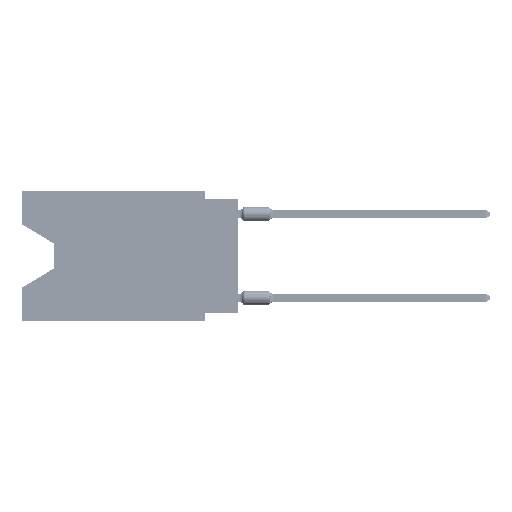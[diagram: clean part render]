
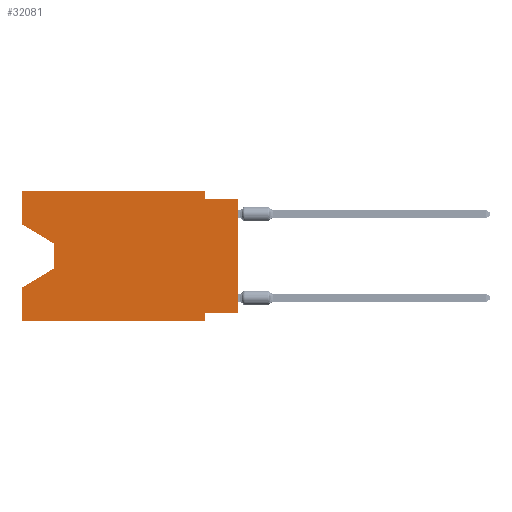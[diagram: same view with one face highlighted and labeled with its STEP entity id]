
A CAD part, left-side view. The second image highlights one B-rep face of the part: STEP entity #32081.
In plain terms, the highlighted planar face has unit normal (-1, 0, 0).
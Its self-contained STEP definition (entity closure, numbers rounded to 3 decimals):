
#15 = CARTESIAN_POINT ( 'NONE',  ( 0., 16.383, -2.546 ) ) ;
#694 = EDGE_CURVE ( 'NONE', #13441, #64532, #63593, .T. ) ;
#866 = VECTOR ( 'NONE', #3840, 1000. ) ;
#1405 = LINE ( 'NONE', #64976, #63932 ) ;
#1498 = DIRECTION ( 'NONE',  ( 0., 1., 0. ) ) ;
#2017 = ORIENTED_EDGE ( 'NONE', *, *, #50201, .F. ) ;
#3273 = ORIENTED_EDGE ( 'NONE', *, *, #44155, .T. ) ;
#3840 = DIRECTION ( 'NONE',  ( 0., 0., -1. ) ) ;
#5650 = DIRECTION ( 'NONE',  ( 0., 0., -1. ) ) ;
#6818 = VERTEX_POINT ( 'NONE', #44249 ) ;
#7020 = CARTESIAN_POINT ( 'NONE',  ( 0., 2.54, 0. ) ) ;
#7268 = CARTESIAN_POINT ( 'NONE',  ( 0., 0., -0.635 ) ) ;
#8455 = ORIENTED_EDGE ( 'NONE', *, *, #694, .T. ) ;
#8976 = VECTOR ( 'NONE', #45054, 1000. ) ;
#9652 = ORIENTED_EDGE ( 'NONE', *, *, #63180, .T. ) ;
#9658 = VERTEX_POINT ( 'NONE', #32526 ) ;
#11703 = DIRECTION ( 'NONE',  ( 0., 0., -1. ) ) ;
#13441 = VERTEX_POINT ( 'NONE', #51184 ) ;
#15927 = VECTOR ( 'NONE', #1498, 1000. ) ;
#16631 = ORIENTED_EDGE ( 'NONE', *, *, #37350, .F. ) ;
#17335 = ORIENTED_EDGE ( 'NONE', *, *, #67220, .F. ) ;
#17505 = LINE ( 'NONE', #7020, #40923 ) ;
#17630 = DIRECTION ( 'NONE',  ( 0., -1., 0. ) ) ;
#18729 = CARTESIAN_POINT ( 'NONE',  ( 0., 0., -0.635 ) ) ;
#19974 = VECTOR ( 'NONE', #42565, 1000. ) ;
#20356 = EDGE_CURVE ( 'NONE', #59912, #29675, #22171, .T. ) ;
#22171 = LINE ( 'NONE', #27079, #57389 ) ;
#23335 = LINE ( 'NONE', #7268, #61497 ) ;
#23520 = VECTOR ( 'NONE', #51082, 1000. ) ;
#23574 = EDGE_CURVE ( 'NONE', #48259, #6818, #59783, .T. ) ;
#24421 = LINE ( 'NONE', #61103, #8976 ) ;
#24930 = VERTEX_POINT ( 'NONE', #28432 ) ;
#25836 = CARTESIAN_POINT ( 'NONE',  ( 0., 13.97, -4.013 ) ) ;
#26499 = LINE ( 'NONE', #58636, #19974 ) ;
#26813 = CARTESIAN_POINT ( 'NONE',  ( 0., 16.383, -7.36 ) ) ;
#27079 = CARTESIAN_POINT ( 'NONE',  ( 0., 16.383, 0. ) ) ;
#27426 = CARTESIAN_POINT ( 'NONE',  ( 0., 2.54, -9.271 ) ) ;
#27497 = VERTEX_POINT ( 'NONE', #41341 ) ;
#27695 = CARTESIAN_POINT ( 'NONE',  ( 0., 0., -9.271 ) ) ;
#28432 = CARTESIAN_POINT ( 'NONE',  ( 0., 2.54, -0.635 ) ) ;
#29599 = ORIENTED_EDGE ( 'NONE', *, *, #56746, .F. ) ;
#29675 = VERTEX_POINT ( 'NONE', #50338 ) ;
#30651 = VERTEX_POINT ( 'NONE', #18729 ) ;
#32081 = ADVANCED_FACE ( 'NONE', ( #33329 ), #64420, .F. ) ;
#32390 = VECTOR ( 'NONE', #53031, 1000. ) ;
#32526 = CARTESIAN_POINT ( 'NONE',  ( 0., 13.97, -5.893 ) ) ;
#33329 = FACE_OUTER_BOUND ( 'NONE', #39149, .T. ) ;
#34933 = DIRECTION ( 'NONE',  ( 0., 0., -1. ) ) ;
#35330 = ORIENTED_EDGE ( 'NONE', *, *, #23574, .F. ) ;
#37350 = EDGE_CURVE ( 'NONE', #48322, #43253, #26499, .T. ) ;
#39149 = EDGE_LOOP ( 'NONE', ( #8455, #64731, #9652, #16631, #3273, #35330, #17335, #54751, #2017, #29599, #65523, #47394 ) ) ;
#39301 = VECTOR ( 'NONE', #53462, 1000. ) ;
#40923 = VECTOR ( 'NONE', #34933, 1000. ) ;
#41341 = CARTESIAN_POINT ( 'NONE',  ( 0., 0., -9.271 ) ) ;
#42565 = DIRECTION ( 'NONE',  ( 0., 0., 1. ) ) ;
#43253 = VERTEX_POINT ( 'NONE', #26813 ) ;
#44155 = EDGE_CURVE ( 'NONE', #48322, #6818, #24421, .T. ) ;
#44249 = CARTESIAN_POINT ( 'NONE',  ( 0., 2.54, -9.906 ) ) ;
#44332 = EDGE_CURVE ( 'NONE', #27497, #30651, #52347, .T. ) ;
#44516 = DIRECTION ( 'NONE',  ( 1., 0., 0. ) ) ;
#45054 = DIRECTION ( 'NONE',  ( 0., -1., 0. ) ) ;
#47394 = ORIENTED_EDGE ( 'NONE', *, *, #66400, .F. ) ;
#48259 = VERTEX_POINT ( 'NONE', #27426 ) ;
#48322 = VERTEX_POINT ( 'NONE', #54993 ) ;
#49310 = AXIS2_PLACEMENT_3D ( 'NONE', #54986, #44516, #11703 ) ;
#50201 = EDGE_CURVE ( 'NONE', #24930, #30651, #23335, .T. ) ;
#50338 = CARTESIAN_POINT ( 'NONE',  ( 0., 2.54, 0. ) ) ;
#50806 = CARTESIAN_POINT ( 'NONE',  ( 0., 13.97, -4.013 ) ) ;
#51082 = DIRECTION ( 'NONE',  ( 0., 0.855, -0.519 ) ) ;
#51184 = CARTESIAN_POINT ( 'NONE',  ( 0., 16.383, -2.546 ) ) ;
#51435 = CARTESIAN_POINT ( 'NONE',  ( 0., 13.97, -5.893 ) ) ;
#52347 = LINE ( 'NONE', #62831, #32390 ) ;
#52383 = LINE ( 'NONE', #25836, #866 ) ;
#53031 = DIRECTION ( 'NONE',  ( 0., 0., 1. ) ) ;
#53462 = DIRECTION ( 'NONE',  ( 0., -0.855, -0.519 ) ) ;
#53672 = CARTESIAN_POINT ( 'NONE',  ( 0., 16.383, 0. ) ) ;
#54189 = CARTESIAN_POINT ( 'NONE',  ( 0., 2.54, -9.906 ) ) ;
#54751 = ORIENTED_EDGE ( 'NONE', *, *, #44332, .T. ) ;
#54986 = CARTESIAN_POINT ( 'NONE',  ( 0., 16.383, 0. ) ) ;
#54993 = CARTESIAN_POINT ( 'NONE',  ( 0., 16.383, -9.906 ) ) ;
#56746 = EDGE_CURVE ( 'NONE', #29675, #24930, #17505, .T. ) ;
#57389 = VECTOR ( 'NONE', #17630, 1000. ) ;
#57691 = LINE ( 'NONE', #51435, #23520 ) ;
#58146 = EDGE_CURVE ( 'NONE', #64532, #9658, #52383, .T. ) ;
#58636 = CARTESIAN_POINT ( 'NONE',  ( 0., 16.383, 0. ) ) ;
#59783 = LINE ( 'NONE', #54189, #65496 ) ;
#59912 = VERTEX_POINT ( 'NONE', #53672 ) ;
#61039 = DIRECTION ( 'NONE',  ( 0., -1., 0. ) ) ;
#61103 = CARTESIAN_POINT ( 'NONE',  ( 0., 16.383, -9.906 ) ) ;
#61497 = VECTOR ( 'NONE', #61039, 1000. ) ;
#62831 = CARTESIAN_POINT ( 'NONE',  ( 0., 0., 0. ) ) ;
#63180 = EDGE_CURVE ( 'NONE', #9658, #43253, #57691, .T. ) ;
#63593 = LINE ( 'NONE', #15, #39301 ) ;
#63932 = VECTOR ( 'NONE', #65315, 1000. ) ;
#64420 = PLANE ( 'NONE',  #49310 ) ;
#64532 = VERTEX_POINT ( 'NONE', #50806 ) ;
#64731 = ORIENTED_EDGE ( 'NONE', *, *, #58146, .T. ) ;
#64976 = CARTESIAN_POINT ( 'NONE',  ( 0., 16.383, 0. ) ) ;
#65315 = DIRECTION ( 'NONE',  ( 0., 0., 1. ) ) ;
#65496 = VECTOR ( 'NONE', #5650, 1000. ) ;
#65523 = ORIENTED_EDGE ( 'NONE', *, *, #20356, .F. ) ;
#65752 = LINE ( 'NONE', #27695, #15927 ) ;
#66400 = EDGE_CURVE ( 'NONE', #13441, #59912, #1405, .T. ) ;
#67220 = EDGE_CURVE ( 'NONE', #27497, #48259, #65752, .T. ) ;
